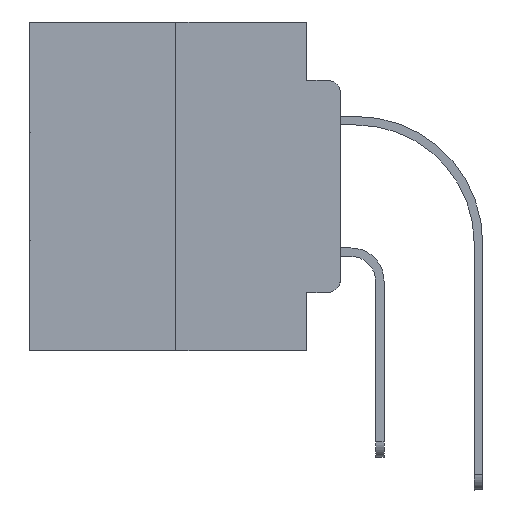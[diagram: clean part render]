
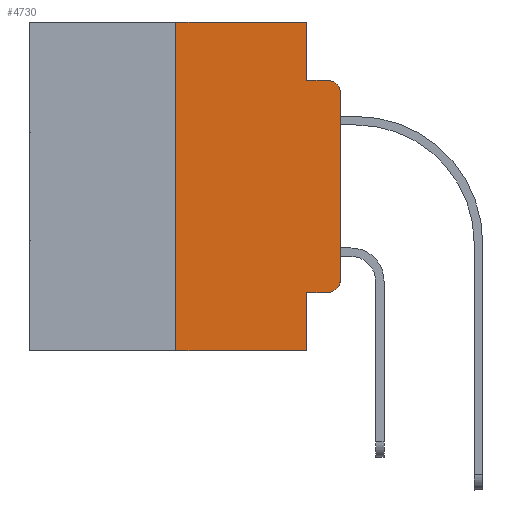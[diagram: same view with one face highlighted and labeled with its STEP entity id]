
A CAD part, left-side view. The second image highlights one B-rep face of the part: STEP entity #4730.
In plain terms, the highlighted planar face has unit normal (-1, 0, 0).
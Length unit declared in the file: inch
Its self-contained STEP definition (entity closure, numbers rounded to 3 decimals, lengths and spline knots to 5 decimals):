
#882 = LINE ( 'NONE', #29578, #21772 ) ;
#1051 = DIRECTION ( 'NONE',  ( 0., -1., 0. ) ) ;
#1854 = EDGE_CURVE ( 'NONE', #3279, #19160, #24937, .T. ) ;
#1991 = ORIENTED_EDGE ( 'NONE', *, *, #14300, .F. ) ;
#2150 = CARTESIAN_POINT ( 'NONE',  ( 0., 0.473, 0. ) ) ;
#2172 = EDGE_CURVE ( 'NONE', #7650, #14217, #25869, .T. ) ;
#2472 = VECTOR ( 'NONE', #29943, 39.37008 ) ;
#2549 = CARTESIAN_POINT ( 'NONE',  ( 0., 0.02, -0.4115 ) ) ;
#2718 = CARTESIAN_POINT ( 'NONE',  ( 0., 0.051, 0. ) ) ;
#3174 = EDGE_LOOP ( 'NONE', ( #12926, #8709, #1991, #28816, #18660, #29997, #18730, #16208, #10330, #4677 ) ) ;
#3199 = VERTEX_POINT ( 'NONE', #2549 ) ;
#3279 = VERTEX_POINT ( 'NONE', #18190 ) ;
#3550 = EDGE_CURVE ( 'NONE', #3199, #3279, #10307, .T. ) ;
#3941 = CARTESIAN_POINT ( 'NONE',  ( 0., 0.051, -0.4115 ) ) ;
#4677 = ORIENTED_EDGE ( 'NONE', *, *, #3550, .T. ) ;
#4730 = ADVANCED_FACE ( 'NONE', ( #5812 ), #6273, .F. ) ;
#4796 = CARTESIAN_POINT ( 'NONE',  ( 0., 0.02, -0.3915 ) ) ;
#5812 = FACE_OUTER_BOUND ( 'NONE', #3174, .T. ) ;
#5921 = EDGE_CURVE ( 'NONE', #8195, #10194, #12544, .T. ) ;
#6273 = PLANE ( 'NONE',  #8355 ) ;
#7650 = VERTEX_POINT ( 'NONE', #19545 ) ;
#7819 = AXIS2_PLACEMENT_3D ( 'NONE', #4796, #14620, #12124 ) ;
#8051 = CARTESIAN_POINT ( 'NONE',  ( 0., 0.051, 0. ) ) ;
#8111 = LINE ( 'NONE', #20416, #2472 ) ;
#8195 = VERTEX_POINT ( 'NONE', #12112 ) ;
#8355 = AXIS2_PLACEMENT_3D ( 'NONE', #27645, #27514, #15492 ) ;
#8709 = ORIENTED_EDGE ( 'NONE', *, *, #18788, .T. ) ;
#9905 = VECTOR ( 'NONE', #21771, 39.37008 ) ;
#10118 = LINE ( 'NONE', #26813, #10397 ) ;
#10130 = CARTESIAN_POINT ( 'NONE',  ( 0., 0., 0. ) ) ;
#10194 = VERTEX_POINT ( 'NONE', #30162 ) ;
#10307 = CIRCLE ( 'NONE', #7819, 0.02 ) ;
#10330 = ORIENTED_EDGE ( 'NONE', *, *, #23435, .T. ) ;
#10397 = VECTOR ( 'NONE', #10567, 39.37008 ) ;
#10567 = DIRECTION ( 'NONE',  ( 0., 0., 1. ) ) ;
#11107 = DIRECTION ( 'NONE',  ( 0., -1., 0. ) ) ;
#11304 = VECTOR ( 'NONE', #29618, 39.37008 ) ;
#11904 = AXIS2_PLACEMENT_3D ( 'NONE', #26070, #23401, #21062 ) ;
#12112 = CARTESIAN_POINT ( 'NONE',  ( 0., 0.051, -0.4115 ) ) ;
#12119 = DIRECTION ( 'NONE',  ( 0., -1., 0. ) ) ;
#12124 = DIRECTION ( 'NONE',  ( 0., 0., -1. ) ) ;
#12544 = LINE ( 'NONE', #2718, #18281 ) ;
#12926 = ORIENTED_EDGE ( 'NONE', *, *, #1854, .T. ) ;
#13760 = EDGE_CURVE ( 'NONE', #18259, #7650, #10118, .T. ) ;
#14217 = VERTEX_POINT ( 'NONE', #8051 ) ;
#14300 = EDGE_CURVE ( 'NONE', #29189, #24174, #26484, .T. ) ;
#14540 = CARTESIAN_POINT ( 'NONE',  ( 0., 0.051, -0.0885 ) ) ;
#14620 = DIRECTION ( 'NONE',  ( -1., 0., 0. ) ) ;
#15492 = DIRECTION ( 'NONE',  ( 0., 0., -1. ) ) ;
#15570 = EDGE_CURVE ( 'NONE', #18259, #10194, #882, .T. ) ;
#16208 = ORIENTED_EDGE ( 'NONE', *, *, #5921, .F. ) ;
#17868 = CIRCLE ( 'NONE', #11904, 0.02 ) ;
#18190 = CARTESIAN_POINT ( 'NONE',  ( 0., 0., -0.3915 ) ) ;
#18259 = VERTEX_POINT ( 'NONE', #28589 ) ;
#18281 = VECTOR ( 'NONE', #29092, 39.37008 ) ;
#18660 = ORIENTED_EDGE ( 'NONE', *, *, #2172, .F. ) ;
#18730 = ORIENTED_EDGE ( 'NONE', *, *, #15570, .T. ) ;
#18788 = EDGE_CURVE ( 'NONE', #19160, #24174, #17868, .T. ) ;
#19160 = VERTEX_POINT ( 'NONE', #20992 ) ;
#19545 = CARTESIAN_POINT ( 'NONE',  ( 0., 0.25, 0. ) ) ;
#19897 = CARTESIAN_POINT ( 'NONE',  ( 0., 0.051, -0.0885 ) ) ;
#20416 = CARTESIAN_POINT ( 'NONE',  ( 0., 0.051, 0. ) ) ;
#20992 = CARTESIAN_POINT ( 'NONE',  ( 0., 0., -0.1085 ) ) ;
#21062 = DIRECTION ( 'NONE',  ( 0., 0., -1. ) ) ;
#21771 = DIRECTION ( 'NONE',  ( 0., -1., 0. ) ) ;
#21772 = VECTOR ( 'NONE', #1051, 39.37008 ) ;
#22795 = LINE ( 'NONE', #3941, #28869 ) ;
#23401 = DIRECTION ( 'NONE',  ( -1., 0., 0. ) ) ;
#23435 = EDGE_CURVE ( 'NONE', #8195, #3199, #22795, .T. ) ;
#24174 = VERTEX_POINT ( 'NONE', #29718 ) ;
#24937 = LINE ( 'NONE', #10130, #11304 ) ;
#25869 = LINE ( 'NONE', #2150, #28991 ) ;
#26070 = CARTESIAN_POINT ( 'NONE',  ( 0., 0.02, -0.1085 ) ) ;
#26484 = LINE ( 'NONE', #19897, #9905 ) ;
#26813 = CARTESIAN_POINT ( 'NONE',  ( 0., 0.25, 0. ) ) ;
#27514 = DIRECTION ( 'NONE',  ( 1., 0., 0. ) ) ;
#27645 = CARTESIAN_POINT ( 'NONE',  ( 0., 0.473, 0. ) ) ;
#28340 = EDGE_CURVE ( 'NONE', #14217, #29189, #8111, .T. ) ;
#28589 = CARTESIAN_POINT ( 'NONE',  ( 0., 0.25, -0.5 ) ) ;
#28816 = ORIENTED_EDGE ( 'NONE', *, *, #28340, .F. ) ;
#28869 = VECTOR ( 'NONE', #11107, 39.37008 ) ;
#28991 = VECTOR ( 'NONE', #12119, 39.37008 ) ;
#29092 = DIRECTION ( 'NONE',  ( 0., 0., -1. ) ) ;
#29189 = VERTEX_POINT ( 'NONE', #14540 ) ;
#29578 = CARTESIAN_POINT ( 'NONE',  ( 0., 0.473, -0.5 ) ) ;
#29618 = DIRECTION ( 'NONE',  ( 0., 0., 1. ) ) ;
#29718 = CARTESIAN_POINT ( 'NONE',  ( 0., 0.02, -0.0885 ) ) ;
#29943 = DIRECTION ( 'NONE',  ( 0., 0., -1. ) ) ;
#29997 = ORIENTED_EDGE ( 'NONE', *, *, #13760, .F. ) ;
#30162 = CARTESIAN_POINT ( 'NONE',  ( 0., 0.051, -0.5 ) ) ;
